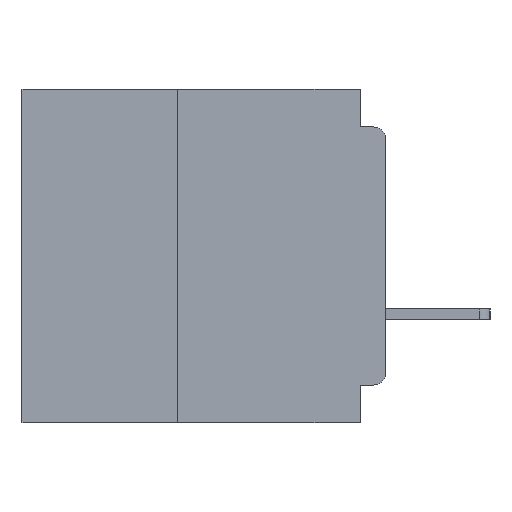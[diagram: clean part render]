
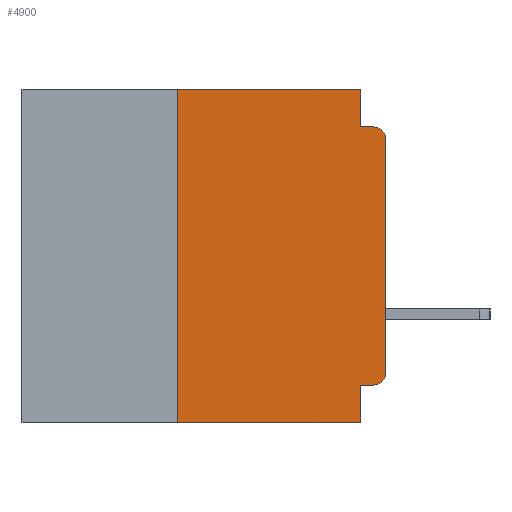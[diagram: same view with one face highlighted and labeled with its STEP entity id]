
A CAD part, left-side view. The second image highlights one B-rep face of the part: STEP entity #4900.
In plain terms, the highlighted planar face has unit normal (-1, 0, 0).
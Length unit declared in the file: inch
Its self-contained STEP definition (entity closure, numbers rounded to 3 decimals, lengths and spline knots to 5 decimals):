
#847 = DIRECTION ( 'NONE',  ( 0., 0., -1. ) ) ;
#949 = DIRECTION ( 'NONE',  ( -1., 0., 0. ) ) ;
#1019 = CARTESIAN_POINT ( 'NONE',  ( 0., 0.015, -0.06 ) ) ;
#1098 = LINE ( 'NONE', #5248, #11514 ) ;
#1110 = CARTESIAN_POINT ( 'NONE',  ( 0., 0.031, -0.4 ) ) ;
#1647 = DIRECTION ( 'NONE',  ( 0., -1., 0. ) ) ;
#4900 = ADVANCED_FACE ( 'NONE', ( #35155 ), #12913, .F. ) ;
#5094 = AXIS2_PLACEMENT_3D ( 'NONE', #1019, #949, #847 ) ;
#5248 = CARTESIAN_POINT ( 'NONE',  ( 0., 0.437, -0.4 ) ) ;
#5251 = EDGE_CURVE ( 'NONE', #32339, #28306, #21140, .T. ) ;
#6298 = VECTOR ( 'NONE', #14707, 39.37008 ) ;
#6892 = LINE ( 'NONE', #21580, #16036 ) ;
#7506 = EDGE_CURVE ( 'NONE', #47166, #9194, #45843, .T. ) ;
#8694 = AXIS2_PLACEMENT_3D ( 'NONE', #13079, #12844, #12795 ) ;
#9100 = VERTEX_POINT ( 'NONE', #35139 ) ;
#9194 = VERTEX_POINT ( 'NONE', #20089 ) ;
#9255 = ORIENTED_EDGE ( 'NONE', *, *, #12758, .T. ) ;
#9415 = VERTEX_POINT ( 'NONE', #32454 ) ;
#10205 = ORIENTED_EDGE ( 'NONE', *, *, #39293, .F. ) ;
#10560 = ORIENTED_EDGE ( 'NONE', *, *, #40208, .T. ) ;
#10680 = VERTEX_POINT ( 'NONE', #28569 ) ;
#11402 = ORIENTED_EDGE ( 'NONE', *, *, #5251, .T. ) ;
#11514 = VECTOR ( 'NONE', #28649, 39.37008 ) ;
#12484 = DIRECTION ( 'NONE',  ( 0., 0., -1. ) ) ;
#12758 = EDGE_CURVE ( 'NONE', #9100, #9194, #1098, .T. ) ;
#12795 = DIRECTION ( 'NONE',  ( 0., 0., -1. ) ) ;
#12844 = DIRECTION ( 'NONE',  ( 1., 0., 0. ) ) ;
#12913 = PLANE ( 'NONE',  #8694 ) ;
#13079 = CARTESIAN_POINT ( 'NONE',  ( 0., 0.437, 0. ) ) ;
#13206 = DIRECTION ( 'NONE',  ( 0., 1., 0. ) ) ;
#14186 = ORIENTED_EDGE ( 'NONE', *, *, #7506, .F. ) ;
#14707 = DIRECTION ( 'NONE',  ( 0., 0., 1. ) ) ;
#15238 = VERTEX_POINT ( 'NONE', #27588 ) ;
#15976 = VECTOR ( 'NONE', #24486, 39.37008 ) ;
#16036 = VECTOR ( 'NONE', #25492, 39.37008 ) ;
#16552 = ORIENTED_EDGE ( 'NONE', *, *, #17994, .F. ) ;
#16857 = CARTESIAN_POINT ( 'NONE',  ( 0., 0.015, -0.34 ) ) ;
#17078 = EDGE_LOOP ( 'NONE', ( #37648, #11402, #10205, #25466, #49445, #16552, #9255, #14186, #28235, #10560 ) ) ;
#17994 = EDGE_CURVE ( 'NONE', #9100, #10680, #27093, .T. ) ;
#19106 = AXIS2_PLACEMENT_3D ( 'NONE', #16857, #44072, #20808 ) ;
#19577 = LINE ( 'NONE', #20171, #28744 ) ;
#20011 = EDGE_CURVE ( 'NONE', #31367, #32339, #20558, .T. ) ;
#20089 = CARTESIAN_POINT ( 'NONE',  ( 0., 0.031, -0.4 ) ) ;
#20148 = CARTESIAN_POINT ( 'NONE',  ( 0., 0., 0. ) ) ;
#20171 = CARTESIAN_POINT ( 'NONE',  ( 0., 0.031, 0. ) ) ;
#20229 = CIRCLE ( 'NONE', #19106, 0.015 ) ;
#20558 = LINE ( 'NONE', #20148, #29734 ) ;
#20808 = DIRECTION ( 'NONE',  ( 0., 0., -1. ) ) ;
#20975 = EDGE_CURVE ( 'NONE', #9415, #47166, #23477, .T. ) ;
#21140 = CIRCLE ( 'NONE', #5094, 0.015 ) ;
#21580 = CARTESIAN_POINT ( 'NONE',  ( 0., 0., -0.045 ) ) ;
#22270 = VECTOR ( 'NONE', #13206, 39.37008 ) ;
#22759 = VERTEX_POINT ( 'NONE', #44674 ) ;
#22900 = CARTESIAN_POINT ( 'NONE',  ( 0., 0., -0.06 ) ) ;
#23214 = EDGE_CURVE ( 'NONE', #15238, #22759, #19577, .T. ) ;
#23477 = LINE ( 'NONE', #44333, #22270 ) ;
#24486 = DIRECTION ( 'NONE',  ( 0., 0., -1. ) ) ;
#25466 = ORIENTED_EDGE ( 'NONE', *, *, #23214, .F. ) ;
#25492 = DIRECTION ( 'NONE',  ( 0., -1., 0. ) ) ;
#27093 = LINE ( 'NONE', #30431, #6298 ) ;
#27588 = CARTESIAN_POINT ( 'NONE',  ( 0., 0.031, 0. ) ) ;
#27835 = DIRECTION ( 'NONE',  ( 0., 0., 1. ) ) ;
#28235 = ORIENTED_EDGE ( 'NONE', *, *, #20975, .F. ) ;
#28306 = VERTEX_POINT ( 'NONE', #34335 ) ;
#28569 = CARTESIAN_POINT ( 'NONE',  ( 0., 0.25, 0. ) ) ;
#28649 = DIRECTION ( 'NONE',  ( 0., -1., 0. ) ) ;
#28744 = VECTOR ( 'NONE', #12484, 39.37008 ) ;
#29734 = VECTOR ( 'NONE', #27835, 39.37008 ) ;
#30431 = CARTESIAN_POINT ( 'NONE',  ( 0., 0.25, -0.4 ) ) ;
#31367 = VERTEX_POINT ( 'NONE', #32105 ) ;
#32105 = CARTESIAN_POINT ( 'NONE',  ( 0., 0., -0.34 ) ) ;
#32339 = VERTEX_POINT ( 'NONE', #22900 ) ;
#32454 = CARTESIAN_POINT ( 'NONE',  ( 0., 0.015, -0.355 ) ) ;
#34335 = CARTESIAN_POINT ( 'NONE',  ( 0., 0.015, -0.045 ) ) ;
#35139 = CARTESIAN_POINT ( 'NONE',  ( 0., 0.25, -0.4 ) ) ;
#35155 = FACE_OUTER_BOUND ( 'NONE', #17078, .T. ) ;
#36244 = VECTOR ( 'NONE', #1647, 39.37008 ) ;
#36654 = CARTESIAN_POINT ( 'NONE',  ( 0., 0.437, 0. ) ) ;
#37648 = ORIENTED_EDGE ( 'NONE', *, *, #20011, .T. ) ;
#39293 = EDGE_CURVE ( 'NONE', #22759, #28306, #6892, .T. ) ;
#40208 = EDGE_CURVE ( 'NONE', #9415, #31367, #20229, .T. ) ;
#41176 = CARTESIAN_POINT ( 'NONE',  ( 0., 0.031, -0.355 ) ) ;
#44072 = DIRECTION ( 'NONE',  ( -1., 0., 0. ) ) ;
#44333 = CARTESIAN_POINT ( 'NONE',  ( 0., 0., -0.355 ) ) ;
#44674 = CARTESIAN_POINT ( 'NONE',  ( 0., 0.031, -0.045 ) ) ;
#45843 = LINE ( 'NONE', #1110, #15976 ) ;
#46544 = LINE ( 'NONE', #36654, #36244 ) ;
#47055 = EDGE_CURVE ( 'NONE', #10680, #15238, #46544, .T. ) ;
#47166 = VERTEX_POINT ( 'NONE', #41176 ) ;
#49445 = ORIENTED_EDGE ( 'NONE', *, *, #47055, .F. ) ;
